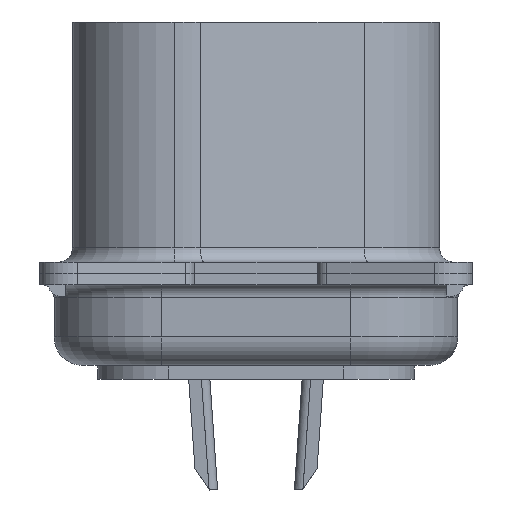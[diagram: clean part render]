
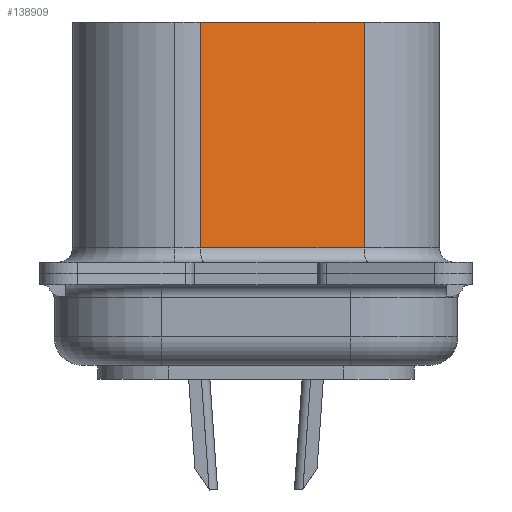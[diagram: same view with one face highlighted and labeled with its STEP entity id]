
A CAD part, left-side view. The second image highlights one B-rep face of the part: STEP entity #138909.
In plain terms, the highlighted planar face has unit normal (-0.966, -0.259, 0).
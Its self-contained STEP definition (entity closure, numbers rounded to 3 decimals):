
#2135 = VERTEX_POINT ( 'NONE', #66004 ) ;
#4049 = DIRECTION ( 'NONE',  ( 0., 0., -1. ) ) ;
#5709 = DIRECTION ( 'NONE',  ( 0.966, 0.259, 0. ) ) ;
#6548 = DIRECTION ( 'NONE',  ( -0.259, 0.966, 0. ) ) ;
#9328 = LINE ( 'NONE', #141689, #16854 ) ;
#14804 = VERTEX_POINT ( 'NONE', #78680 ) ;
#15177 = LINE ( 'NONE', #121114, #23022 ) ;
#16854 = VECTOR ( 'NONE', #74246, 1000. ) ;
#23022 = VECTOR ( 'NONE', #4049, 1000. ) ;
#31126 = DIRECTION ( 'NONE',  ( 0., 0., -1. ) ) ;
#35935 = CARTESIAN_POINT ( 'NONE',  ( 6.467, -3.832, 9.3 ) ) ;
#43190 = CARTESIAN_POINT ( 'NONE',  ( 6.467, -3.832, 1.3 ) ) ;
#51891 = VECTOR ( 'NONE', #31126, 1000. ) ;
#52815 = AXIS2_PLACEMENT_3D ( 'NONE', #59507, #5709, #6548 ) ;
#55445 = ORIENTED_EDGE ( 'NONE', *, *, #159906, .T. ) ;
#56140 = FACE_OUTER_BOUND ( 'NONE', #163383, .T. ) ;
#59507 = CARTESIAN_POINT ( 'NONE',  ( 6.467, -3.832, 9.3 ) ) ;
#64295 = CARTESIAN_POINT ( 'NONE',  ( 6.467, -3.832, 1.3 ) ) ;
#66004 = CARTESIAN_POINT ( 'NONE',  ( 4.913, 1.968, 1.3 ) ) ;
#69813 = EDGE_CURVE ( 'NONE', #14804, #166208, #9328, .T. ) ;
#74246 = DIRECTION ( 'NONE',  ( 0.259, -0.966, 0. ) ) ;
#75447 = LINE ( 'NONE', #64295, #94401 ) ;
#78680 = CARTESIAN_POINT ( 'NONE',  ( 4.913, 1.968, 9.3 ) ) ;
#80050 = VERTEX_POINT ( 'NONE', #43190 ) ;
#94401 = VECTOR ( 'NONE', #154858, 1000. ) ;
#97548 = EDGE_CURVE ( 'NONE', #166208, #80050, #152952, .T. ) ;
#99534 = EDGE_CURVE ( 'NONE', #2135, #80050, #75447, .T. ) ;
#104681 = CARTESIAN_POINT ( 'NONE',  ( 6.467, -3.832, 9.3 ) ) ;
#121114 = CARTESIAN_POINT ( 'NONE',  ( 4.913, 1.968, 9.3 ) ) ;
#122766 = PLANE ( 'NONE',  #52815 ) ;
#136230 = ORIENTED_EDGE ( 'NONE', *, *, #97548, .F. ) ;
#138909 = ADVANCED_FACE ( 'NONE', ( #56140 ), #122766, .F. ) ;
#141689 = CARTESIAN_POINT ( 'NONE',  ( 6.467, -3.832, 9.3 ) ) ;
#146969 = ORIENTED_EDGE ( 'NONE', *, *, #69813, .F. ) ;
#152952 = LINE ( 'NONE', #35935, #51891 ) ;
#154724 = ORIENTED_EDGE ( 'NONE', *, *, #99534, .T. ) ;
#154858 = DIRECTION ( 'NONE',  ( 0.259, -0.966, 0. ) ) ;
#159906 = EDGE_CURVE ( 'NONE', #14804, #2135, #15177, .T. ) ;
#163383 = EDGE_LOOP ( 'NONE', ( #55445, #154724, #136230, #146969 ) ) ;
#166208 = VERTEX_POINT ( 'NONE', #104681 ) ;
